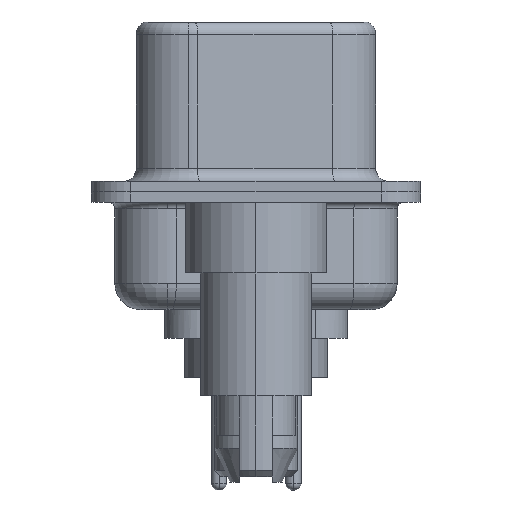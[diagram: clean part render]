
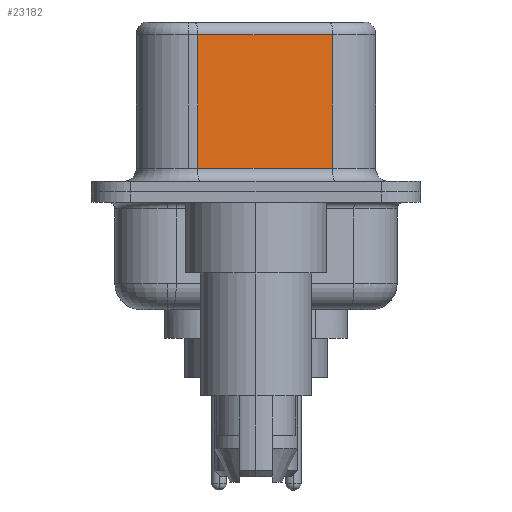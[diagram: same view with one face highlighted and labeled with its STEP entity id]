
A CAD part, left-side view. The second image highlights one B-rep face of the part: STEP entity #23182.
In plain terms, the highlighted planar face has unit normal (-0.985, -0.174, 0).
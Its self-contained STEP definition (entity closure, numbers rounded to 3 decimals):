
#503 = PLANE ( 'NONE',  #7383 ) ;
#803 = FACE_OUTER_BOUND ( 'NONE', #19343, .T. ) ;
#1660 = LINE ( 'NONE', #19330, #15489 ) ;
#2213 = ORIENTED_EDGE ( 'NONE', *, *, #18940, .T. ) ;
#3491 = LINE ( 'NONE', #21691, #21477 ) ;
#4299 = LINE ( 'NONE', #16408, #7525 ) ;
#4703 = VECTOR ( 'NONE', #15414, 1000. ) ;
#4860 = CARTESIAN_POINT ( 'NONE',  ( 4.585, -2.927, 6.02 ) ) ;
#5157 = CARTESIAN_POINT ( 'NONE',  ( 4.585, -2.927, 0.9 ) ) ;
#6147 = VERTEX_POINT ( 'NONE', #4860 ) ;
#7383 = AXIS2_PLACEMENT_3D ( 'NONE', #17651, #19521, #23377 ) ;
#7525 = VECTOR ( 'NONE', #8839, 1000. ) ;
#7623 = VERTEX_POINT ( 'NONE', #19248 ) ;
#7679 = CARTESIAN_POINT ( 'NONE',  ( 3.675, 2.233, 0.9 ) ) ;
#8833 = LINE ( 'NONE', #5157, #4703 ) ;
#8839 = DIRECTION ( 'NONE',  ( -0.174, 0.985, 0. ) ) ;
#9979 = DIRECTION ( 'NONE',  ( 0., 0., -1. ) ) ;
#10450 = ORIENTED_EDGE ( 'NONE', *, *, #15092, .T. ) ;
#15092 = EDGE_CURVE ( 'NONE', #16327, #7623, #8833, .T. ) ;
#15159 = CARTESIAN_POINT ( 'NONE',  ( 3.675, 2.233, 6.02 ) ) ;
#15414 = DIRECTION ( 'NONE',  ( 0.174, -0.985, 0. ) ) ;
#15489 = VECTOR ( 'NONE', #9979, 1000. ) ;
#16327 = VERTEX_POINT ( 'NONE', #7679 ) ;
#16408 = CARTESIAN_POINT ( 'NONE',  ( 4.585, -2.927, 6.02 ) ) ;
#17059 = ORIENTED_EDGE ( 'NONE', *, *, #23207, .T. ) ;
#17651 = CARTESIAN_POINT ( 'NONE',  ( 4.585, -2.927, 6.52 ) ) ;
#17700 = VERTEX_POINT ( 'NONE', #15159 ) ;
#18940 = EDGE_CURVE ( 'NONE', #6147, #17700, #4299, .T. ) ;
#19248 = CARTESIAN_POINT ( 'NONE',  ( 4.585, -2.927, 0.9 ) ) ;
#19330 = CARTESIAN_POINT ( 'NONE',  ( 4.585, -2.927, 6.52 ) ) ;
#19343 = EDGE_LOOP ( 'NONE', ( #21595, #2213, #17059, #10450 ) ) ;
#19521 = DIRECTION ( 'NONE',  ( 0.985, 0.174, 0. ) ) ;
#21074 = EDGE_CURVE ( 'NONE', #6147, #7623, #1660, .T. ) ;
#21477 = VECTOR ( 'NONE', #23878, 1000. ) ;
#21595 = ORIENTED_EDGE ( 'NONE', *, *, #21074, .F. ) ;
#21691 = CARTESIAN_POINT ( 'NONE',  ( 3.675, 2.233, 6.52 ) ) ;
#23182 = ADVANCED_FACE ( 'NONE', ( #803 ), #503, .F. ) ;
#23207 = EDGE_CURVE ( 'NONE', #17700, #16327, #3491, .T. ) ;
#23377 = DIRECTION ( 'NONE',  ( -0.174, 0.985, 0. ) ) ;
#23878 = DIRECTION ( 'NONE',  ( 0., 0., -1. ) ) ;
